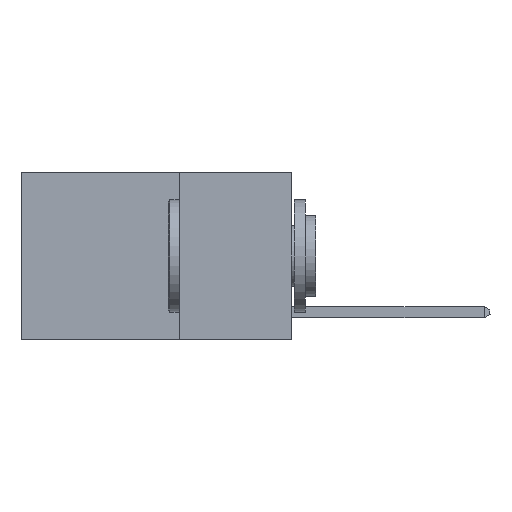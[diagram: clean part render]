
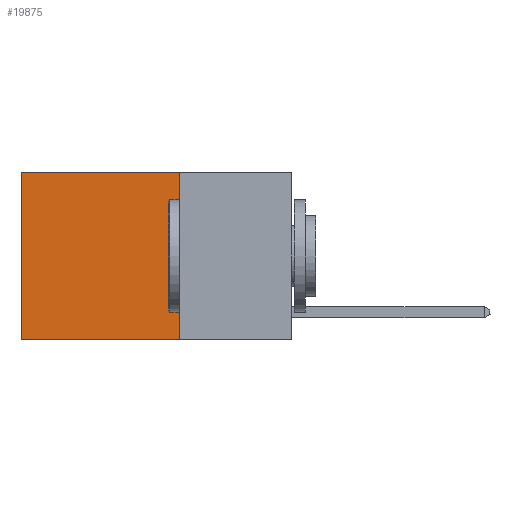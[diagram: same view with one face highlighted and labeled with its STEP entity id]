
A CAD part, left-side view. The second image highlights one B-rep face of the part: STEP entity #19875.
In plain terms, the highlighted planar face has unit normal (-1, 0, 0).
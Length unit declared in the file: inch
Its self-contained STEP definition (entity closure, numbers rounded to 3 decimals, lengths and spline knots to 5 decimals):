
#886 = DIRECTION ( 'NONE',  ( 0., 0., -1. ) ) ;
#1438 = DIRECTION ( 'NONE',  ( 0., 1., 0. ) ) ;
#2524 = LINE ( 'NONE', #4478, #11513 ) ;
#2574 = DIRECTION ( 'NONE',  ( 0., 0., -1. ) ) ;
#2696 = CARTESIAN_POINT ( 'NONE',  ( 0.2625, 0.25, 0. ) ) ;
#3262 = AXIS2_PLACEMENT_3D ( 'NONE', #2696, #23477, #886 ) ;
#4478 = CARTESIAN_POINT ( 'NONE',  ( 0.2625, 0.6, 0. ) ) ;
#6160 = EDGE_LOOP ( 'NONE', ( #25285, #23709, #19435, #18127 ) ) ;
#7637 = CARTESIAN_POINT ( 'NONE',  ( 0.2625, 0.25, 0. ) ) ;
#8420 = CARTESIAN_POINT ( 'NONE',  ( 0.2625, 0.25, 0. ) ) ;
#9074 = LINE ( 'NONE', #21172, #20630 ) ;
#9310 = LINE ( 'NONE', #16165, #21107 ) ;
#11513 = VECTOR ( 'NONE', #24114, 39.37008 ) ;
#12022 = VERTEX_POINT ( 'NONE', #24245 ) ;
#13575 = PLANE ( 'NONE',  #3262 ) ;
#14067 = VERTEX_POINT ( 'NONE', #15338 ) ;
#14215 = VERTEX_POINT ( 'NONE', #19511 ) ;
#14900 = FACE_OUTER_BOUND ( 'NONE', #6160, .T. ) ;
#15338 = CARTESIAN_POINT ( 'NONE',  ( 0.2625, 0.6, -0.37 ) ) ;
#16165 = CARTESIAN_POINT ( 'NONE',  ( 0.2625, 0.25, 0. ) ) ;
#16694 = EDGE_CURVE ( 'NONE', #22582, #12022, #9310, .T. ) ;
#18127 = ORIENTED_EDGE ( 'NONE', *, *, #16694, .T. ) ;
#18176 = VECTOR ( 'NONE', #2574, 39.37008 ) ;
#19435 = ORIENTED_EDGE ( 'NONE', *, *, #19783, .F. ) ;
#19439 = EDGE_CURVE ( 'NONE', #14215, #14067, #9074, .T. ) ;
#19511 = CARTESIAN_POINT ( 'NONE',  ( 0.2625, 0.25, -0.37 ) ) ;
#19783 = EDGE_CURVE ( 'NONE', #22582, #14215, #22195, .T. ) ;
#19875 = ADVANCED_FACE ( 'NONE', ( #14900 ), #13575, .F. ) ;
#20630 = VECTOR ( 'NONE', #1438, 39.37008 ) ;
#21107 = VECTOR ( 'NONE', #24111, 39.37008 ) ;
#21172 = CARTESIAN_POINT ( 'NONE',  ( 0.2625, 0.25, -0.37 ) ) ;
#22195 = LINE ( 'NONE', #8420, #18176 ) ;
#22582 = VERTEX_POINT ( 'NONE', #7637 ) ;
#23477 = DIRECTION ( 'NONE',  ( 1., 0., 0. ) ) ;
#23709 = ORIENTED_EDGE ( 'NONE', *, *, #19439, .F. ) ;
#24111 = DIRECTION ( 'NONE',  ( 0., 1., 0. ) ) ;
#24114 = DIRECTION ( 'NONE',  ( 0., 0., -1. ) ) ;
#24230 = EDGE_CURVE ( 'NONE', #12022, #14067, #2524, .T. ) ;
#24245 = CARTESIAN_POINT ( 'NONE',  ( 0.2625, 0.6, 0. ) ) ;
#25285 = ORIENTED_EDGE ( 'NONE', *, *, #24230, .T. ) ;
